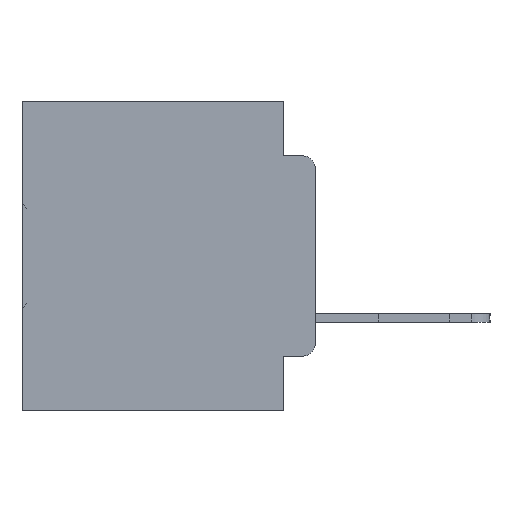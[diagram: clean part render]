
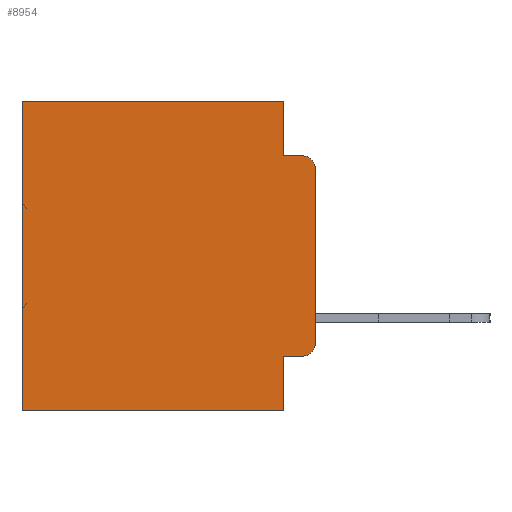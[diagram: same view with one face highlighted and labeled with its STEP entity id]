
A CAD part, left-side view. The second image highlights one B-rep face of the part: STEP entity #8954.
In plain terms, the highlighted planar face has unit normal (-1, 0, 0).
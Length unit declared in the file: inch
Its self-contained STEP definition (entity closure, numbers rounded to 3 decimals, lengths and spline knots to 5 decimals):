
#282 = ORIENTED_EDGE ( 'NONE', *, *, #30893, .T. ) ;
#1274 = ORIENTED_EDGE ( 'NONE', *, *, #24018, .T. ) ;
#1310 = CARTESIAN_POINT ( 'NONE',  ( 0.298, 0.473, 0. ) ) ;
#1648 = LINE ( 'NONE', #16294, #16156 ) ;
#1663 = VECTOR ( 'NONE', #4844, 39.37008 ) ;
#2320 = CARTESIAN_POINT ( 'NONE',  ( 0.298, 0., 0. ) ) ;
#2380 = EDGE_LOOP ( 'NONE', ( #26191, #32995, #12828, #13715, #28575, #7854, #16230, #23332, #282, #1274 ) ) ;
#2438 = DIRECTION ( 'NONE',  ( 0., 1., 0. ) ) ;
#2499 = CARTESIAN_POINT ( 'NONE',  ( 0.298, 0.02, -0.0885 ) ) ;
#2611 = VECTOR ( 'NONE', #33042, 39.37008 ) ;
#2647 = EDGE_CURVE ( 'NONE', #19995, #17880, #18735, .T. ) ;
#3167 = CARTESIAN_POINT ( 'NONE',  ( 0.298, 0.473, -0.5 ) ) ;
#4508 = VERTEX_POINT ( 'NONE', #12377 ) ;
#4844 = DIRECTION ( 'NONE',  ( 0., 0., -1. ) ) ;
#5104 = LINE ( 'NONE', #23696, #19256 ) ;
#5419 = DIRECTION ( 'NONE',  ( 0., -1., 0. ) ) ;
#5936 = EDGE_CURVE ( 'NONE', #23341, #16023, #9042, .T. ) ;
#7854 = ORIENTED_EDGE ( 'NONE', *, *, #12544, .T. ) ;
#8459 = EDGE_CURVE ( 'NONE', #17880, #24135, #11924, .T. ) ;
#8676 = CARTESIAN_POINT ( 'NONE',  ( 0.298, 0.02, -0.3915 ) ) ;
#8954 = ADVANCED_FACE ( 'NONE', ( #26527 ), #24596, .F. ) ;
#9042 = LINE ( 'NONE', #2320, #17340 ) ;
#9760 = CARTESIAN_POINT ( 'NONE',  ( 0.298, 0.051, -0.0885 ) ) ;
#9988 = DIRECTION ( 'NONE',  ( -1., 0., 0. ) ) ;
#10685 = CARTESIAN_POINT ( 'NONE',  ( 0.298, 0.473, 0. ) ) ;
#11005 = VECTOR ( 'NONE', #5419, 39.37008 ) ;
#11608 = DIRECTION ( 'NONE',  ( 0., 0., -1. ) ) ;
#11924 = LINE ( 'NONE', #16823, #18322 ) ;
#12377 = CARTESIAN_POINT ( 'NONE',  ( 0.298, 0.02, -0.4115 ) ) ;
#12418 = DIRECTION ( 'NONE',  ( 0., 0., -1. ) ) ;
#12544 = EDGE_CURVE ( 'NONE', #21736, #24135, #24100, .T. ) ;
#12828 = ORIENTED_EDGE ( 'NONE', *, *, #30269, .F. ) ;
#13511 = VERTEX_POINT ( 'NONE', #9760 ) ;
#13551 = CARTESIAN_POINT ( 'NONE',  ( 0.298, 0.051, 0. ) ) ;
#13715 = ORIENTED_EDGE ( 'NONE', *, *, #18017, .F. ) ;
#13974 = DIRECTION ( 'NONE',  ( 1., 0., 0. ) ) ;
#14385 = CARTESIAN_POINT ( 'NONE',  ( 0.298, 0.051, -0.4115 ) ) ;
#16023 = VERTEX_POINT ( 'NONE', #22919 ) ;
#16156 = VECTOR ( 'NONE', #19017, 39.37008 ) ;
#16230 = ORIENTED_EDGE ( 'NONE', *, *, #8459, .F. ) ;
#16254 = EDGE_CURVE ( 'NONE', #35399, #21736, #5104, .T. ) ;
#16294 = CARTESIAN_POINT ( 'NONE',  ( 0.298, 0.051, 0. ) ) ;
#16653 = AXIS2_PLACEMENT_3D ( 'NONE', #26208, #9988, #28747 ) ;
#16823 = CARTESIAN_POINT ( 'NONE',  ( 0.298, 0., -0.5 ) ) ;
#17340 = VECTOR ( 'NONE', #12418, 39.37008 ) ;
#17880 = VERTEX_POINT ( 'NONE', #31165 ) ;
#18017 = EDGE_CURVE ( 'NONE', #35399, #13511, #1648, .T. ) ;
#18322 = VECTOR ( 'NONE', #2438, 39.37008 ) ;
#18735 = LINE ( 'NONE', #13551, #2611 ) ;
#18740 = VERTEX_POINT ( 'NONE', #2499 ) ;
#19017 = DIRECTION ( 'NONE',  ( 0., 0., -1. ) ) ;
#19256 = VECTOR ( 'NONE', #21017, 39.37008 ) ;
#19482 = CARTESIAN_POINT ( 'NONE',  ( 0.298, 0.051, -0.4115 ) ) ;
#19995 = VERTEX_POINT ( 'NONE', #14385 ) ;
#21017 = DIRECTION ( 'NONE',  ( 0., 1., 0. ) ) ;
#21736 = VERTEX_POINT ( 'NONE', #1310 ) ;
#22547 = LINE ( 'NONE', #31499, #35357 ) ;
#22865 = AXIS2_PLACEMENT_3D ( 'NONE', #8676, #27599, #11608 ) ;
#22919 = CARTESIAN_POINT ( 'NONE',  ( 0.298, 0., -0.3915 ) ) ;
#23332 = ORIENTED_EDGE ( 'NONE', *, *, #2647, .F. ) ;
#23341 = VERTEX_POINT ( 'NONE', #31484 ) ;
#23696 = CARTESIAN_POINT ( 'NONE',  ( 0.298, 0., 0. ) ) ;
#24018 = EDGE_CURVE ( 'NONE', #4508, #16023, #30779, .T. ) ;
#24100 = LINE ( 'NONE', #10685, #1663 ) ;
#24135 = VERTEX_POINT ( 'NONE', #3167 ) ;
#24469 = CIRCLE ( 'NONE', #16653, 0.02 ) ;
#24596 = PLANE ( 'NONE',  #31107 ) ;
#25269 = CARTESIAN_POINT ( 'NONE',  ( 0.298, 0.051, 0. ) ) ;
#26152 = LINE ( 'NONE', #19482, #11005 ) ;
#26191 = ORIENTED_EDGE ( 'NONE', *, *, #5936, .F. ) ;
#26208 = CARTESIAN_POINT ( 'NONE',  ( 0.298, 0.02, -0.1085 ) ) ;
#26527 = FACE_OUTER_BOUND ( 'NONE', #2380, .T. ) ;
#27599 = DIRECTION ( 'NONE',  ( -1., 0., 0. ) ) ;
#28575 = ORIENTED_EDGE ( 'NONE', *, *, #16254, .T. ) ;
#28747 = DIRECTION ( 'NONE',  ( 0., 0., -1. ) ) ;
#29722 = CARTESIAN_POINT ( 'NONE',  ( 0.298, 0., 0. ) ) ;
#30269 = EDGE_CURVE ( 'NONE', #13511, #18740, #22547, .T. ) ;
#30779 = CIRCLE ( 'NONE', #22865, 0.02 ) ;
#30893 = EDGE_CURVE ( 'NONE', #19995, #4508, #26152, .T. ) ;
#31107 = AXIS2_PLACEMENT_3D ( 'NONE', #29722, #13974, #32317 ) ;
#31165 = CARTESIAN_POINT ( 'NONE',  ( 0.298, 0.051, -0.5 ) ) ;
#31484 = CARTESIAN_POINT ( 'NONE',  ( 0.298, 0., -0.1085 ) ) ;
#31499 = CARTESIAN_POINT ( 'NONE',  ( 0.298, 0.051, -0.0885 ) ) ;
#32003 = EDGE_CURVE ( 'NONE', #23341, #18740, #24469, .T. ) ;
#32317 = DIRECTION ( 'NONE',  ( 0., 0., -1. ) ) ;
#32995 = ORIENTED_EDGE ( 'NONE', *, *, #32003, .T. ) ;
#33042 = DIRECTION ( 'NONE',  ( 0., 0., -1. ) ) ;
#34058 = DIRECTION ( 'NONE',  ( 0., -1., 0. ) ) ;
#35357 = VECTOR ( 'NONE', #34058, 39.37008 ) ;
#35399 = VERTEX_POINT ( 'NONE', #25269 ) ;
